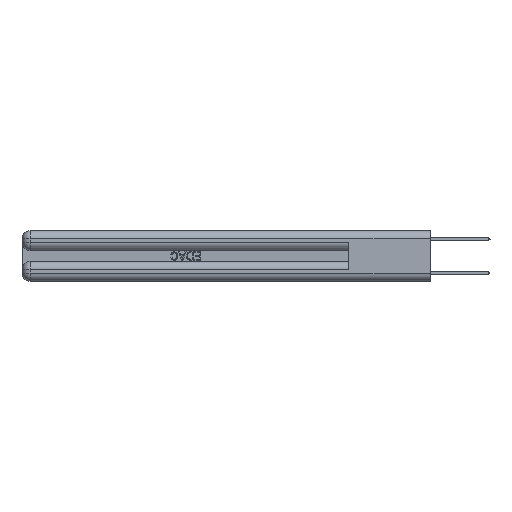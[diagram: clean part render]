
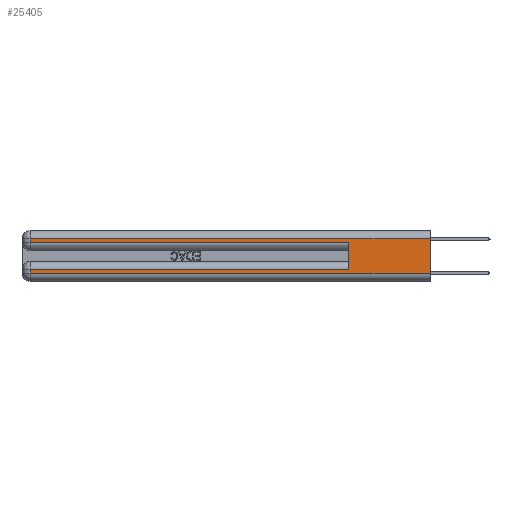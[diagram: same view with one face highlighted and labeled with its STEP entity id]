
A CAD part, left-side view. The second image highlights one B-rep face of the part: STEP entity #25405.
In plain terms, the highlighted planar face has unit normal (-1, 0, 0).
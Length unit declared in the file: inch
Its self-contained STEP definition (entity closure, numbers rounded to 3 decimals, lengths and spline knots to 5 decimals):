
#891 = DIRECTION ( 'NONE',  ( 0., -1., 0. ) ) ;
#1319 = VERTEX_POINT ( 'NONE', #8146 ) ;
#2252 = CARTESIAN_POINT ( 'NONE',  ( 0., 2.94, 0.085 ) ) ;
#2260 = ORIENTED_EDGE ( 'NONE', *, *, #2516, .T. ) ;
#2516 = EDGE_CURVE ( 'NONE', #10616, #1319, #24266, .T. ) ;
#2946 = EDGE_CURVE ( 'NONE', #21882, #16182, #31021, .T. ) ;
#2957 = VECTOR ( 'NONE', #23770, 39.37008 ) ;
#3268 = CARTESIAN_POINT ( 'NONE',  ( 0., 0., 0.37 ) ) ;
#3930 = CARTESIAN_POINT ( 'NONE',  ( 0., 0., 0.285 ) ) ;
#4094 = LINE ( 'NONE', #6339, #31318 ) ;
#4485 = ORIENTED_EDGE ( 'NONE', *, *, #9737, .F. ) ;
#4839 = EDGE_CURVE ( 'NONE', #4930, #16182, #8949, .T. ) ;
#4930 = VERTEX_POINT ( 'NONE', #12336 ) ;
#6198 = CARTESIAN_POINT ( 'NONE',  ( 0., 0., 0.06 ) ) ;
#6339 = CARTESIAN_POINT ( 'NONE',  ( 0., 0.6, 0.145 ) ) ;
#7706 = CARTESIAN_POINT ( 'NONE',  ( 0., 0., 0.31 ) ) ;
#7715 = DIRECTION ( 'NONE',  ( 0., 1., 0. ) ) ;
#7889 = DIRECTION ( 'NONE',  ( 0., -1., 0. ) ) ;
#8146 = CARTESIAN_POINT ( 'NONE',  ( 0., 2.94, 0.285 ) ) ;
#8259 = ORIENTED_EDGE ( 'NONE', *, *, #4839, .T. ) ;
#8949 = LINE ( 'NONE', #10393, #20142 ) ;
#9174 = VERTEX_POINT ( 'NONE', #12000 ) ;
#9381 = DIRECTION ( 'NONE',  ( 0., 0., 1. ) ) ;
#9737 = EDGE_CURVE ( 'NONE', #9174, #26169, #4094, .T. ) ;
#10154 = ORIENTED_EDGE ( 'NONE', *, *, #30376, .T. ) ;
#10393 = CARTESIAN_POINT ( 'NONE',  ( 0., 0., 0.06 ) ) ;
#10616 = VERTEX_POINT ( 'NONE', #13608 ) ;
#10644 = VECTOR ( 'NONE', #27962, 39.37008 ) ;
#11803 = ORIENTED_EDGE ( 'NONE', *, *, #25637, .T. ) ;
#11980 = PLANE ( 'NONE',  #26665 ) ;
#12000 = CARTESIAN_POINT ( 'NONE',  ( 0., 0.6, 0.085 ) ) ;
#12096 = DIRECTION ( 'NONE',  ( 0., 0., -1. ) ) ;
#12336 = CARTESIAN_POINT ( 'NONE',  ( 0., 2.94, 0.06 ) ) ;
#13608 = CARTESIAN_POINT ( 'NONE',  ( 0., 2.94, 0.31 ) ) ;
#14365 = FACE_OUTER_BOUND ( 'NONE', #15552, .T. ) ;
#14425 = VERTEX_POINT ( 'NONE', #2252 ) ;
#14888 = LINE ( 'NONE', #30438, #32503 ) ;
#15552 = EDGE_LOOP ( 'NONE', ( #28662, #11803, #2260, #18509, #4485, #10154, #25328, #8259 ) ) ;
#15645 = EDGE_CURVE ( 'NONE', #14425, #4930, #24722, .T. ) ;
#16182 = VERTEX_POINT ( 'NONE', #6198 ) ;
#18509 = ORIENTED_EDGE ( 'NONE', *, *, #25262, .T. ) ;
#19822 = DIRECTION ( 'NONE',  ( 1., 0., 0. ) ) ;
#20142 = VECTOR ( 'NONE', #7889, 39.37008 ) ;
#20273 = CARTESIAN_POINT ( 'NONE',  ( 0., 2.94, 0.37 ) ) ;
#20332 = LINE ( 'NONE', #7706, #32373 ) ;
#20359 = LINE ( 'NONE', #3930, #21138 ) ;
#21138 = VECTOR ( 'NONE', #891, 39.37008 ) ;
#21882 = VERTEX_POINT ( 'NONE', #26972 ) ;
#23770 = DIRECTION ( 'NONE',  ( 0., 0., -1. ) ) ;
#23922 = VECTOR ( 'NONE', #27789, 39.37008 ) ;
#24266 = LINE ( 'NONE', #20273, #10644 ) ;
#24722 = LINE ( 'NONE', #27347, #23922 ) ;
#25262 = EDGE_CURVE ( 'NONE', #1319, #26169, #20359, .T. ) ;
#25328 = ORIENTED_EDGE ( 'NONE', *, *, #15645, .T. ) ;
#25405 = ADVANCED_FACE ( 'NONE', ( #14365 ), #11980, .F. ) ;
#25637 = EDGE_CURVE ( 'NONE', #21882, #10616, #20332, .T. ) ;
#26169 = VERTEX_POINT ( 'NONE', #28330 ) ;
#26665 = AXIS2_PLACEMENT_3D ( 'NONE', #26929, #19822, #12096 ) ;
#26929 = CARTESIAN_POINT ( 'NONE',  ( 0., 0., 0.37 ) ) ;
#26972 = CARTESIAN_POINT ( 'NONE',  ( 0., 0., 0.31 ) ) ;
#27347 = CARTESIAN_POINT ( 'NONE',  ( 0., 2.94, 0.37 ) ) ;
#27789 = DIRECTION ( 'NONE',  ( 0., 0., -1. ) ) ;
#27962 = DIRECTION ( 'NONE',  ( 0., 0., -1. ) ) ;
#28330 = CARTESIAN_POINT ( 'NONE',  ( 0., 0.6, 0.285 ) ) ;
#28363 = DIRECTION ( 'NONE',  ( 0., 1., 0. ) ) ;
#28662 = ORIENTED_EDGE ( 'NONE', *, *, #2946, .F. ) ;
#30376 = EDGE_CURVE ( 'NONE', #9174, #14425, #14888, .T. ) ;
#30438 = CARTESIAN_POINT ( 'NONE',  ( 0., 0., 0.085 ) ) ;
#31021 = LINE ( 'NONE', #3268, #2957 ) ;
#31318 = VECTOR ( 'NONE', #9381, 39.37008 ) ;
#32373 = VECTOR ( 'NONE', #28363, 39.37008 ) ;
#32503 = VECTOR ( 'NONE', #7715, 39.37008 ) ;
